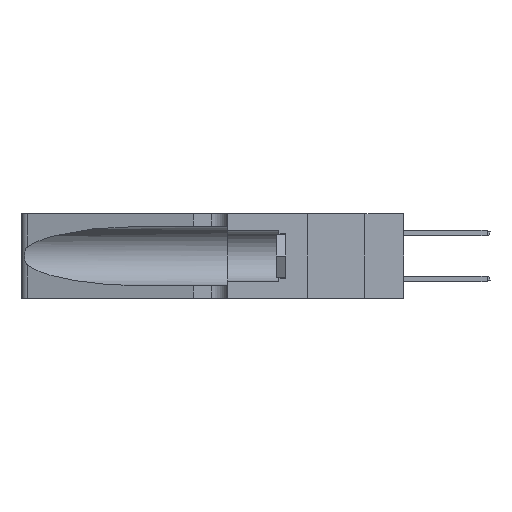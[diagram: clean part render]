
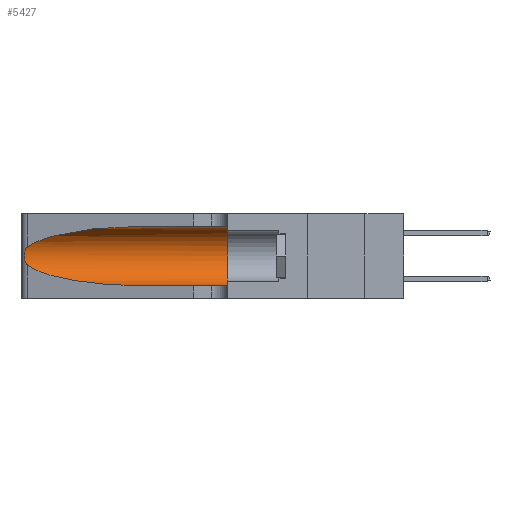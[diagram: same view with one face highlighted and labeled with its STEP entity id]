
A CAD part, left-side view. The second image highlights one B-rep face of the part: STEP entity #5427.
In plain terms, the highlighted cylindrical face has radius 3.308 mm (diameter 6.617 mm), a partial arc.
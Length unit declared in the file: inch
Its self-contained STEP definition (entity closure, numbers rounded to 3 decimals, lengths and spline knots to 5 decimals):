
#240 = CARTESIAN_POINT ( 'NONE',  ( 0.1305, 0.35, 0.31525 ) ) ;
#241 = VECTOR ( 'NONE', #10582, 39.37008 ) ;
#1511 = EDGE_CURVE ( 'NONE', #26742, #14455, #14047, .T. ) ;
#2056 = CARTESIAN_POINT ( 'NONE',  ( 0.26075, 1.23896, 0.19203 ) ) ;
#2306 = CARTESIAN_POINT ( 'NONE',  ( 0.26018, 1.23835, 0.19895 ) ) ;
#2413 = CARTESIAN_POINT ( 'NONE',  ( 0.26075, 1.23896, 0.178 ) ) ;
#2576 = CARTESIAN_POINT ( 'NONE',  ( 0.1305, 1.61858, 0.185 ) ) ;
#2807 = FACE_OUTER_BOUND ( 'NONE', #15697, .T. ) ;
#3219 = CARTESIAN_POINT ( 'NONE',  ( 0.25487, 1.22718, 0.14631 ) ) ;
#4875 = CARTESIAN_POINT ( 'NONE',  ( 0.25787, 1.23484, 0.2124 ) ) ;
#5120 = CARTESIAN_POINT ( 'NONE',  ( 0.1305, 0.72297, 0.31525 ) ) ;
#5357 = CARTESIAN_POINT ( 'NONE',  ( 0.1305, 0.35, 0.05475 ) ) ;
#5427 = ADVANCED_FACE ( 'NONE', ( #2807 ), #29192, .F. ) ;
#5612 = CARTESIAN_POINT ( 'NONE',  ( 0.25487, 1.22718, 0.14631 ) ) ;
#7287 = CARTESIAN_POINT ( 'NONE',  ( 0.25639, 1.23184, 0.21858 ) ) ;
#8031 = LINE ( 'NONE', #27164, #16881 ) ;
#9531 = CARTESIAN_POINT ( 'NONE',  ( 0.25487, 1.22718, 0.22369 ) ) ;
#10246 = CARTESIAN_POINT ( 'NONE',  ( 0.25854, 1.2359, 0.20912 ) ) ;
#10582 = DIRECTION ( 'NONE',  ( 0., -1., 0. ) ) ;
#10945 = CARTESIAN_POINT ( 'NONE',  ( 0.2373, 1.15595, 0.08982 ) ) ;
#11026 = DIRECTION ( 'NONE',  ( 0., -1., 0. ) ) ;
#11581 = CARTESIAN_POINT ( 'NONE',  ( 0.1305, 0.35, 0.185 ) ) ;
#12091 = EDGE_CURVE ( 'NONE', #14455, #32428, #28171, .T. ) ;
#12260 = CARTESIAN_POINT ( 'NONE',  ( 0.25555, 1.22994, 0.2215 ) ) ;
#12347 = ORIENTED_EDGE ( 'NONE', *, *, #1511, .T. ) ;
#13551 = VERTEX_POINT ( 'NONE', #5357 ) ;
#13928 = CARTESIAN_POINT ( 'NONE',  ( 0.25487, 1.22718, 0.22369 ) ) ;
#14047 =( BOUNDED_CURVE ( )  B_SPLINE_CURVE ( 3, ( #28137, #31172, #17735, #23119 ),
 .UNSPECIFIED., .F., .F. ) 
 B_SPLINE_CURVE_WITH_KNOTS ( ( 4, 4 ),
 ( 1.5708, 2.84003 ),
 .UNSPECIFIED. ) 
 CURVE ( )  GEOMETRIC_REPRESENTATION_ITEM ( )  RATIONAL_B_SPLINE_CURVE ( ( 1., 0.87, 0.87, 1. ) ) 
 REPRESENTATION_ITEM ( '' )  );
#14278 = DIRECTION ( 'NONE',  ( 0., 0., 1. ) ) ;
#14455 = VERTEX_POINT ( 'NONE', #13928 ) ;
#15697 = EDGE_LOOP ( 'NONE', ( #12347, #29507, #25761, #24516, #32615, #19244 ) ) ;
#16565 = CARTESIAN_POINT ( 'NONE',  ( 0.18966, 0.96281, 0.05475 ) ) ;
#16881 = VECTOR ( 'NONE', #11026, 39.37008 ) ;
#17735 = CARTESIAN_POINT ( 'NONE',  ( 0.2373, 1.15595, 0.28018 ) ) ;
#18130 = CARTESIAN_POINT ( 'NONE',  ( 0.1305, 0.72297, 0.05475 ) ) ;
#18797 = CARTESIAN_POINT ( 'NONE',  ( 0.26017, 1.23833, 0.17102 ) ) ;
#18910 = EDGE_CURVE ( 'NONE', #32428, #20693, #22011, .T. ) ;
#18915 = AXIS2_PLACEMENT_3D ( 'NONE', #11581, #22165, #14278 ) ;
#19244 = ORIENTED_EDGE ( 'NONE', *, *, #27213, .F. ) ;
#19460 = VERTEX_POINT ( 'NONE', #240 ) ;
#20693 = VERTEX_POINT ( 'NONE', #18130 ) ;
#20769 = LINE ( 'NONE', #26615, #241 ) ;
#20803 = EDGE_CURVE ( 'NONE', #20693, #13551, #8031, .T. ) ;
#20849 = DIRECTION ( 'NONE',  ( 0., -1., 0. ) ) ;
#21512 = CARTESIAN_POINT ( 'NONE',  ( 0.25789, 1.23486, 0.15765 ) ) ;
#22011 =( BOUNDED_CURVE ( )  B_SPLINE_CURVE ( 3, ( #3219, #10945, #16565, #22097 ),
 .UNSPECIFIED., .F., .F. ) 
 B_SPLINE_CURVE_WITH_KNOTS ( ( 4, 4 ),
 ( 3.44316, 4.71239 ),
 .UNSPECIFIED. ) 
 CURVE ( )  GEOMETRIC_REPRESENTATION_ITEM ( )  RATIONAL_B_SPLINE_CURVE ( ( 1., 0.87, 0.87, 1. ) ) 
 REPRESENTATION_ITEM ( '' )  );
#22097 = CARTESIAN_POINT ( 'NONE',  ( 0.1305, 0.72297, 0.05475 ) ) ;
#22165 = DIRECTION ( 'NONE',  ( 0., 1., 0. ) ) ;
#22269 = EDGE_CURVE ( 'NONE', #19460, #13551, #29733, .T. ) ;
#23119 = CARTESIAN_POINT ( 'NONE',  ( 0.25487, 1.22718, 0.22369 ) ) ;
#24436 = CARTESIAN_POINT ( 'NONE',  ( 0.25856, 1.23593, 0.16098 ) ) ;
#24516 = ORIENTED_EDGE ( 'NONE', *, *, #20803, .T. ) ;
#25761 = ORIENTED_EDGE ( 'NONE', *, *, #18910, .T. ) ;
#26615 = CARTESIAN_POINT ( 'NONE',  ( 0.1305, 1.61858, 0.31525 ) ) ;
#26628 = CARTESIAN_POINT ( 'NONE',  ( 0.25555, 1.22993, 0.14849 ) ) ;
#26742 = VERTEX_POINT ( 'NONE', #5120 ) ;
#26863 = CARTESIAN_POINT ( 'NONE',  ( 0.25487, 1.22718, 0.14631 ) ) ;
#27099 = CARTESIAN_POINT ( 'NONE',  ( 0.25639, 1.23186, 0.15144 ) ) ;
#27164 = CARTESIAN_POINT ( 'NONE',  ( 0.1305, 1.61858, 0.05475 ) ) ;
#27213 = EDGE_CURVE ( 'NONE', #26742, #19460, #20769, .T. ) ;
#28137 = CARTESIAN_POINT ( 'NONE',  ( 0.1305, 0.72297, 0.31525 ) ) ;
#28171 = B_SPLINE_CURVE_WITH_KNOTS ( 'NONE', 3,
 ( #9531, #12260, #7287, #4875, #10246, #2306, #2056, #2413, #18797, #24436, #21512, #27099, #26628, #26863 ),
 .UNSPECIFIED., .F., .F.,
 ( 4, 2, 2, 2, 2, 2, 4 ),
 ( 0., 0.00027, 0.00053, 0.00107, 0.0016, 0.00187, 0.00214 ),
 .UNSPECIFIED. ) ;
#29136 = DIRECTION ( 'NONE',  ( 0., 0., -1. ) ) ;
#29192 = CYLINDRICAL_SURFACE ( 'NONE', #32774, 0.13025 ) ;
#29507 = ORIENTED_EDGE ( 'NONE', *, *, #12091, .T. ) ;
#29733 = CIRCLE ( 'NONE', #18915, 0.13025 ) ;
#31172 = CARTESIAN_POINT ( 'NONE',  ( 0.18966, 0.96281, 0.31525 ) ) ;
#32428 = VERTEX_POINT ( 'NONE', #5612 ) ;
#32615 = ORIENTED_EDGE ( 'NONE', *, *, #22269, .F. ) ;
#32774 = AXIS2_PLACEMENT_3D ( 'NONE', #2576, #20849, #29136 ) ;
